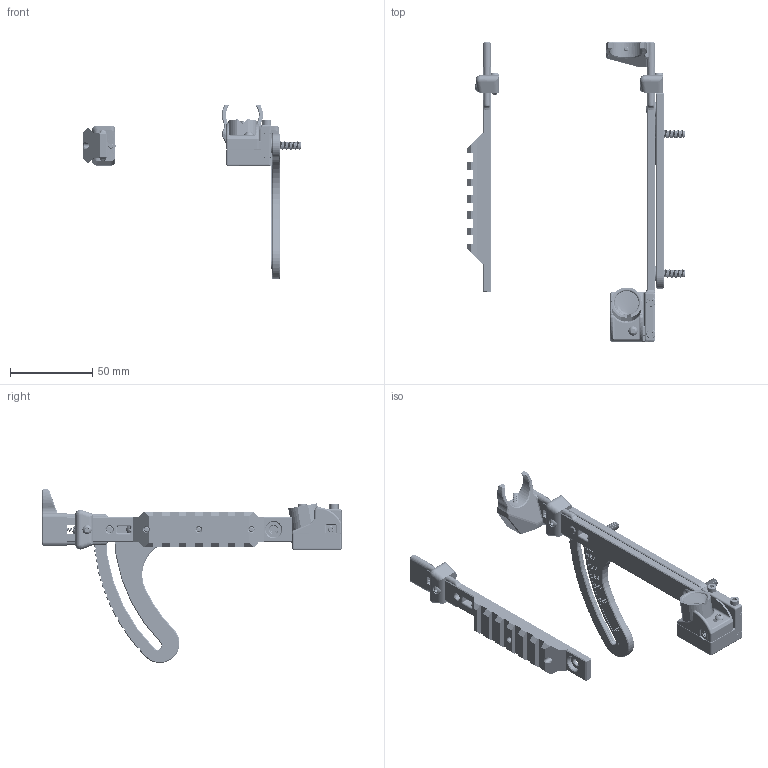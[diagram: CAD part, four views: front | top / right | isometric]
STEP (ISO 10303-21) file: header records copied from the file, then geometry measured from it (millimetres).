
FILE_DESCRIPTION(/* description */ (''),/* implementation_level */ '2;1');
FILE_NAME(/* name */ 'JP Launcher Quadrant Sight.step',/* time_stamp */ '2022-08-15T19:42:10-04:00',/* author */ (''),/* organization */ (''),/* preprocessor_version */ 'ST-DEVELOPER v19',/* originating_system */ 'Autodesk Translation Framework v11.7.0.108',/* authorisation */ '');
FILE_SCHEMA (('AUTOMOTIVE_DESIGN { 1 0 10303 214 3 1 1 }'));
Products named in the file (44): Balls Quad Sight; RH Quadrant Sight; Quadrant Scale; Diopter Range Arm; Slide; M3x12 BHCS (Sharpened) 91239A117_Button Head Hex Drive Screw; M3x8 BHCS 91239A113_Button Head Hex Drive Screw; Hardware (1); M3x20 SHCS 91274A109_Zinc-Aluminum-Coated Alloy Steel Socket Head Scr
ew; M3 Threaded Insert (1)^X Carriage Frame_X Carriage (1); 3mmx15mm spring (Pen) 8969T194_316 Stainless Steel Corrosion-Resistan
t Compression Springs; M5x20 BHCS 91239A233_Button Head Hex Drive Screw; M5x8 BHCS 91239A222_Button Head Hex Drive Screw; M5x15 BHCS 92095A127_Button Head Hex Drive Screw; Range Arm (1); Rear Sight; Hardware; M3 Threaded Insert (1)^X Carriage Frame_X Carriage; M3 Threaded Insert (1)^X Carriage Frame_X Carriage (2); M3x8 SHCS or BHCS 91290A113_Alloy Steel Socket Head Screw; M3x10 BHCS 91239A113_Button Head Hex Drive Screw; 3mm Washer 94744A711_Zinc-Plated Steel Washer for Soft Material; M3 Threaded Insert (1)^X Carriage Frame_X Carriage (3); M3 Threaded Insert (1)^X Carriage Frame_X Carriage (4); M3 Threaded Insert (1)^X Carriage Frame_X Carriage (4) (1); M3x25 SHCS 91274A111_Zinc-Aluminum-Coated Alloy Steel Socket Head Scr
ew; M3x25 SHCS 91274A111_Zinc-Aluminum-Coated Alloy Steel Socket Head Scr
ew (1); M3x15 BHCS 91239A811_Button Head Hex Drive Screw; Drum Slide; Drum; Rear Sight Base (1); Picatinny Range Arm; Slide (1); M3x12 BHCS (Sharpened) 91239A117_Button Head Hex Drive Screw (1); M3x8 BHCS 91239A113_Button Head Hex Drive Screw (1); 3mmx15mm spring (Pen) 8969T194_316 Stainless Steel Corrosion-Resistan
t Compression Springs (1) (1); Range Arm (1) (1); Rail Section; m3x8 BHCS 97763A813_18-8 Stainless Steel Button Head Hex Drive Screws; m3X8 BHCS 97763A813_18-8 Stainless Steel Button Head Hex Drive Screws
 (1) ...
Assembly tree (44 placements, depth 5):
  Balls Quad Sight
    RH Quadrant Sight
      Quadrant Scale
    Diopter Range Arm
      Slide
        M3x12 BHCS (Sharpened) 91239A117_Button Head Hex Drive Screw
        M3x8 BHCS 91239A113_Button Head Hex Drive Screw
      Hardware (1)
        M3x20 SHCS 91274A109_Zinc-Aluminum-Coated Alloy Steel Socket Head Scr
ew
        M3 Threaded Insert (1)^X Carriage Frame_X Carriage (1)
        3mmx15mm spring (Pen) 8969T194_316 Stainless Steel Corrosion-Resistan
t Compression Springs
        M5x20 BHCS 91239A233_Button Head Hex Drive Screw
        M5x8 BHCS 91239A222_Button Head Hex Drive Screw
        M5x15 BHCS 92095A127_Button Head Hex Drive Screw
      Range Arm (1)
      Rear Sight
        Hardware
          M3 Threaded Insert (1)^X Carriage Frame_X Carriage
          M3 Threaded Insert (1)^X Carriage Frame_X Carriage (2)
          M3x8 SHCS or BHCS 91290A113_Alloy Steel Socket Head Screw
          M3x10 BHCS 91239A113_Button Head Hex Drive Screw
          3mm Washer 94744A711_Zinc-Plated Steel Washer for Soft Material  x2
          M3 Threaded Insert (1)^X Carriage Frame_X Carriage (3)
          M3 Threaded Insert (1)^X Carriage Frame_X Carriage (4)
          M3 Threaded Insert (1)^X Carriage Frame_X Carriage (4) (1)
          M3x25 SHCS 91274A111_Zinc-Aluminum-Coated Alloy Steel Socket Head Scr
ew
          M3x25 SHCS 91274A111_Zinc-Aluminum-Coated Alloy Steel Socket Head Scr
ew (1)
          M3x15 BHCS 91239A811_Button Head Hex Drive Screw
        Drum Slide
        Drum
        Rear Sight Base (1)
    Picatinny Range Arm
      Slide (1)
        M3x12 BHCS (Sharpened) 91239A117_Button Head Hex Drive Screw (1)
        M3x8 BHCS 91239A113_Button Head Hex Drive Screw (1)
        3mmx15mm spring (Pen) 8969T194_316 Stainless Steel Corrosion-Resistan
t Compression Springs (1) (1)
      Range Arm (1) (1)
      Rail Section
        m3x8 BHCS 97763A813_18-8 Stainless Steel Button Head Hex Drive Screws
        m3X8 BHCS 97763A813_18-8 Stainless Steel Button Head Hex Drive Screws
 (1)
        m3X8 BHCS97763A813_18-8 Stainless Steel Button Head Hex Drive Screws 
(1) (1)
        M3 Threaded Insert (1)^X Carriage Frame_X Carriage (1) (3)
        M3 Threaded Insert (1)^X Carriage Frame_X Carriage (1) (3) (1)
        M3 Threaded Insert (1)^X Carriage Frame_X Carriage (1) (3) (1) (1)
Bounding box: 132.41 x 182.3 x 105.94 mm (x, y, z)
Volume: 74531.8 mm3; surface area: 55284 mm2
Topology: 49 solids, 49 shells, 3881 faces, 10344 edges, 6771 vertices
Faces by surface type: cylinder 1275, bspline 1218, plane 1066, cone 267, torus 35, sphere 20
Full cylindrical faces by diameter (mm): 1.5 x3, 1.75 x4, 1.8 x8, 2 x1, 2.35 x278, 2.5 x11, 2.9 x9, 3 x288, 3.1 x6, 3.2 x7, 3.5 x2, 3.961 x46, 4 x6, 4.2 x19, 4.25 x12, 4.6 x9, 5 x53, 5.1 x1, 5.5 x4, 5.7 x12, 6 x1, 6.8 x2, 8 x1, 8.2 x1, 9.5 x7
Entity records: 221818 total; most frequent: CARTESIAN_POINT 132388, ORIENTED_EDGE 20660, DIRECTION 15043, EDGE_CURVE 10330, VERTEX_POINT 6767, AXIS2_PLACEMENT_3D 5709, EDGE_LOOP 4213, FACE_OUTER_BOUND 3877
